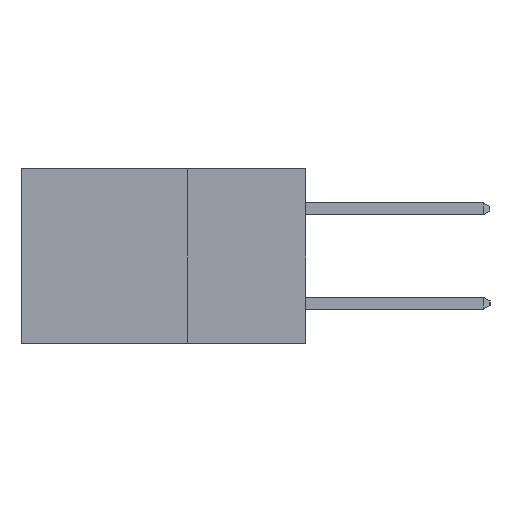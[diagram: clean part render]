
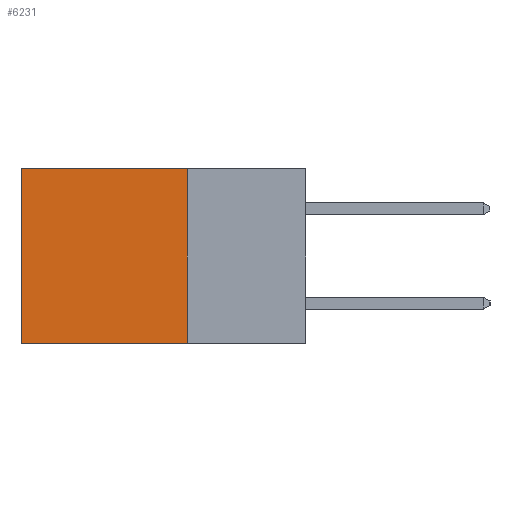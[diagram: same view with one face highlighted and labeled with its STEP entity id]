
A CAD part, left-side view. The second image highlights one B-rep face of the part: STEP entity #6231.
In plain terms, the highlighted planar face has unit normal (-1, 0, 0).
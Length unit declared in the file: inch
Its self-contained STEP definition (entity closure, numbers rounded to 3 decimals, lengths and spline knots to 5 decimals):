
#50 = VERTEX_POINT ( 'NONE', #15982 ) ;
#1005 = VECTOR ( 'NONE', #12010, 39.37008 ) ;
#1310 = CARTESIAN_POINT ( 'NONE',  ( 0.2615, 0.25, -0.37 ) ) ;
#1828 = ORIENTED_EDGE ( 'NONE', *, *, #2460, .F. ) ;
#2460 = EDGE_CURVE ( 'NONE', #9799, #4831, #15305, .T. ) ;
#3616 = LINE ( 'NONE', #4983, #11602 ) ;
#3799 = ORIENTED_EDGE ( 'NONE', *, *, #5271, .T. ) ;
#4168 = EDGE_LOOP ( 'NONE', ( #3799, #7583, #1828, #11326 ) ) ;
#4541 = CARTESIAN_POINT ( 'NONE',  ( 0.2615, 0.25, -0.37 ) ) ;
#4831 = VERTEX_POINT ( 'NONE', #1310 ) ;
#4983 = CARTESIAN_POINT ( 'NONE',  ( 0.2615, 0.25, 0. ) ) ;
#5271 = EDGE_CURVE ( 'NONE', #15908, #50, #5493, .T. ) ;
#5486 = AXIS2_PLACEMENT_3D ( 'NONE', #4541, #6122, #17278 ) ;
#5493 = LINE ( 'NONE', #13545, #1005 ) ;
#6054 = CARTESIAN_POINT ( 'NONE',  ( 0.2615, 0.25, -0.37 ) ) ;
#6122 = DIRECTION ( 'NONE',  ( 1., 0., 0. ) ) ;
#6231 = ADVANCED_FACE ( 'NONE', ( #9656 ), #15677, .F. ) ;
#6559 = DIRECTION ( 'NONE',  ( 0., 1., 0. ) ) ;
#7583 = ORIENTED_EDGE ( 'NONE', *, *, #20603, .F. ) ;
#9074 = EDGE_CURVE ( 'NONE', #9799, #15908, #3616, .T. ) ;
#9656 = FACE_OUTER_BOUND ( 'NONE', #4168, .T. ) ;
#9799 = VERTEX_POINT ( 'NONE', #16113 ) ;
#11326 = ORIENTED_EDGE ( 'NONE', *, *, #9074, .T. ) ;
#11602 = VECTOR ( 'NONE', #6559, 39.37008 ) ;
#11766 = LINE ( 'NONE', #6054, #20160 ) ;
#11905 = CARTESIAN_POINT ( 'NONE',  ( 0.2615, 0.25, -0.37 ) ) ;
#12010 = DIRECTION ( 'NONE',  ( 0., 0., -1. ) ) ;
#13545 = CARTESIAN_POINT ( 'NONE',  ( 0.2615, 0.6, -0.37 ) ) ;
#14821 = VECTOR ( 'NONE', #18212, 39.37008 ) ;
#15305 = LINE ( 'NONE', #11905, #14821 ) ;
#15677 = PLANE ( 'NONE',  #5486 ) ;
#15908 = VERTEX_POINT ( 'NONE', #20198 ) ;
#15982 = CARTESIAN_POINT ( 'NONE',  ( 0.2615, 0.6, -0.37 ) ) ;
#16113 = CARTESIAN_POINT ( 'NONE',  ( 0.2615, 0.25, 0. ) ) ;
#17278 = DIRECTION ( 'NONE',  ( 0., 0., -1. ) ) ;
#18212 = DIRECTION ( 'NONE',  ( 0., 0., -1. ) ) ;
#20160 = VECTOR ( 'NONE', #20315, 39.37008 ) ;
#20198 = CARTESIAN_POINT ( 'NONE',  ( 0.2615, 0.6, 0. ) ) ;
#20315 = DIRECTION ( 'NONE',  ( 0., 1., 0. ) ) ;
#20603 = EDGE_CURVE ( 'NONE', #4831, #50, #11766, .T. ) ;
